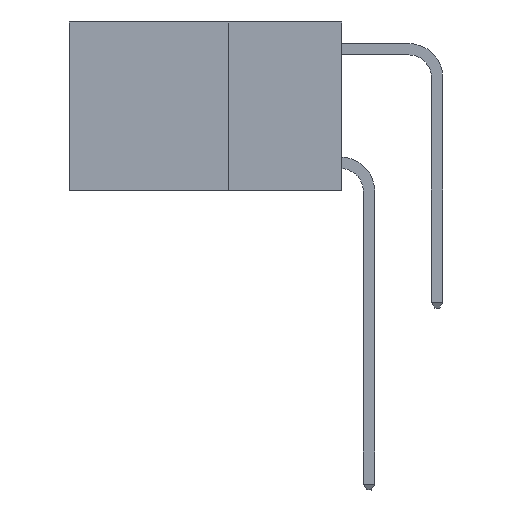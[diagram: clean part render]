
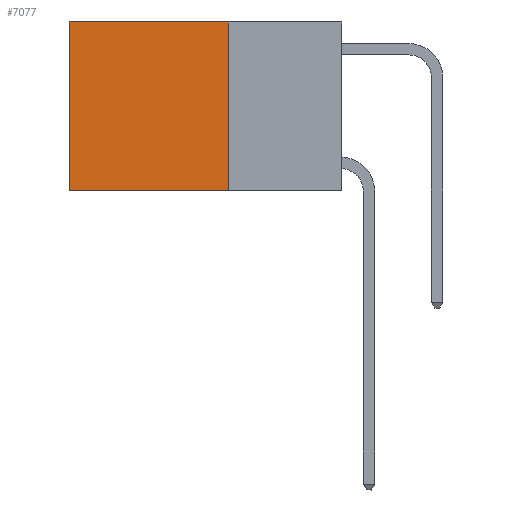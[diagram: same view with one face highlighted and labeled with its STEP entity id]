
A CAD part, left-side view. The second image highlights one B-rep face of the part: STEP entity #7077.
In plain terms, the highlighted planar face has unit normal (-1, 0, 0).
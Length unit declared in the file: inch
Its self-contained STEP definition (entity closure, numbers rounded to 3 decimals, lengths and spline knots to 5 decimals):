
#640 = VERTEX_POINT ( 'NONE', #7663 ) ;
#746 = CARTESIAN_POINT ( 'NONE',  ( 0.2625, 0.25, 0. ) ) ;
#758 = LINE ( 'NONE', #1879, #5044 ) ;
#1343 = VECTOR ( 'NONE', #5728, 39.37008 ) ;
#1417 = CARTESIAN_POINT ( 'NONE',  ( 0.2625, 0.6, -0.37 ) ) ;
#1879 = CARTESIAN_POINT ( 'NONE',  ( 0.2625, 0.25, 0. ) ) ;
#2797 = EDGE_CURVE ( 'NONE', #8819, #6195, #758, .T. ) ;
#2909 = LINE ( 'NONE', #5850, #1343 ) ;
#3322 = CARTESIAN_POINT ( 'NONE',  ( 0.2625, 0.25, -0.37 ) ) ;
#3667 = LINE ( 'NONE', #3322, #6010 ) ;
#4026 = VECTOR ( 'NONE', #8105, 39.37008 ) ;
#4175 = LINE ( 'NONE', #9186, #4026 ) ;
#4808 = EDGE_CURVE ( 'NONE', #6195, #12269, #3667, .T. ) ;
#5044 = VECTOR ( 'NONE', #10880, 39.37008 ) ;
#5728 = DIRECTION ( 'NONE',  ( 0., 0., -1. ) ) ;
#5827 = PLANE ( 'NONE',  #7233 ) ;
#5850 = CARTESIAN_POINT ( 'NONE',  ( 0.2625, 0.6, 0. ) ) ;
#6010 = VECTOR ( 'NONE', #12384, 39.37008 ) ;
#6195 = VERTEX_POINT ( 'NONE', #8853 ) ;
#7073 = ORIENTED_EDGE ( 'NONE', *, *, #8408, .T. ) ;
#7077 = ADVANCED_FACE ( 'NONE', ( #11960 ), #5827, .F. ) ;
#7233 = AXIS2_PLACEMENT_3D ( 'NONE', #9993, #9824, #12754 ) ;
#7663 = CARTESIAN_POINT ( 'NONE',  ( 0.2625, 0.6, 0. ) ) ;
#8105 = DIRECTION ( 'NONE',  ( 0., 1., 0. ) ) ;
#8408 = EDGE_CURVE ( 'NONE', #8819, #640, #4175, .T. ) ;
#8819 = VERTEX_POINT ( 'NONE', #746 ) ;
#8853 = CARTESIAN_POINT ( 'NONE',  ( 0.2625, 0.25, -0.37 ) ) ;
#9186 = CARTESIAN_POINT ( 'NONE',  ( 0.2625, 0.25, 0. ) ) ;
#9243 = EDGE_CURVE ( 'NONE', #640, #12269, #2909, .T. ) ;
#9362 = ORIENTED_EDGE ( 'NONE', *, *, #4808, .F. ) ;
#9824 = DIRECTION ( 'NONE',  ( 1., 0., 0. ) ) ;
#9993 = CARTESIAN_POINT ( 'NONE',  ( 0.2625, 0.25, 0. ) ) ;
#10819 = EDGE_LOOP ( 'NONE', ( #11061, #9362, #10826, #7073 ) ) ;
#10826 = ORIENTED_EDGE ( 'NONE', *, *, #2797, .F. ) ;
#10880 = DIRECTION ( 'NONE',  ( 0., 0., -1. ) ) ;
#11061 = ORIENTED_EDGE ( 'NONE', *, *, #9243, .T. ) ;
#11960 = FACE_OUTER_BOUND ( 'NONE', #10819, .T. ) ;
#12269 = VERTEX_POINT ( 'NONE', #1417 ) ;
#12384 = DIRECTION ( 'NONE',  ( 0., 1., 0. ) ) ;
#12754 = DIRECTION ( 'NONE',  ( 0., 0., -1. ) ) ;
